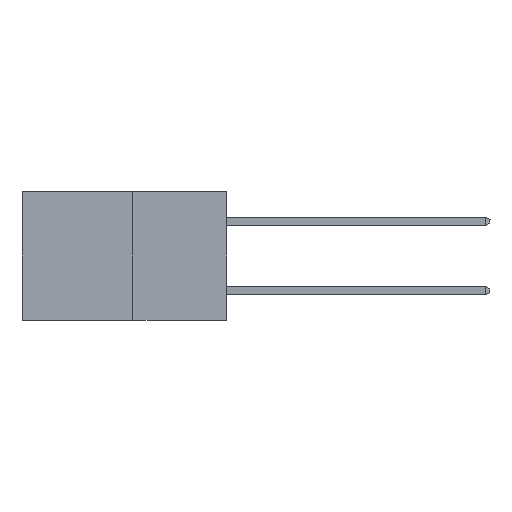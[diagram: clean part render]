
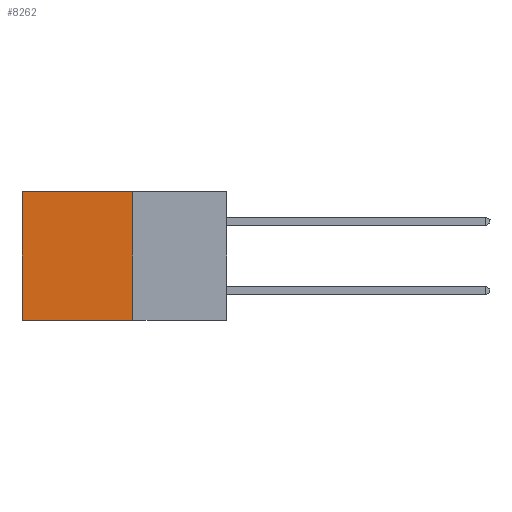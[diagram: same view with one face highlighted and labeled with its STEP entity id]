
A CAD part, left-side view. The second image highlights one B-rep face of the part: STEP entity #8262.
In plain terms, the highlighted planar face has unit normal (-1, 0, 0).
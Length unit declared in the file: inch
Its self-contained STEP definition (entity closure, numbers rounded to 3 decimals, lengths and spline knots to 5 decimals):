
#86 = ORIENTED_EDGE ( 'NONE', *, *, #1455, .T. ) ;
#117 = ORIENTED_EDGE ( 'NONE', *, *, #8861, .F. ) ;
#128 = ORIENTED_EDGE ( 'NONE', *, *, #6020, .F. ) ;
#151 = ORIENTED_EDGE ( 'NONE', *, *, #6541, .T. ) ;
#422 = DIRECTION ( 'NONE',  ( 0., 0., -1. ) ) ;
#516 = CARTESIAN_POINT ( 'NONE',  ( 0.277, 0.59, -0.37 ) ) ;
#811 = FACE_OUTER_BOUND ( 'NONE', #1362, .T. ) ;
#1362 = EDGE_LOOP ( 'NONE', ( #86, #117, #128, #151 ) ) ;
#1455 = EDGE_CURVE ( 'NONE', #7280, #6824, #5242, .T. ) ;
#1714 = CARTESIAN_POINT ( 'NONE',  ( 0.277, 0.27, -0.37 ) ) ;
#1797 = VERTEX_POINT ( 'NONE', #8245 ) ;
#2055 = LINE ( 'NONE', #5171, #2312 ) ;
#2056 = VERTEX_POINT ( 'NONE', #5790 ) ;
#2312 = VECTOR ( 'NONE', #7397, 39.37008 ) ;
#2597 = CARTESIAN_POINT ( 'NONE',  ( 0.277, 0.27, -0.37 ) ) ;
#3045 = DIRECTION ( 'NONE',  ( 0., 1., 0. ) ) ;
#3148 = VECTOR ( 'NONE', #422, 39.37008 ) ;
#3418 = DIRECTION ( 'NONE',  ( 0., 0., -1. ) ) ;
#4685 = LINE ( 'NONE', #1714, #8366 ) ;
#5171 = CARTESIAN_POINT ( 'NONE',  ( 0.277, 0.27, -0.37 ) ) ;
#5242 = LINE ( 'NONE', #516, #3148 ) ;
#5641 = VECTOR ( 'NONE', #3045, 39.37008 ) ;
#5790 = CARTESIAN_POINT ( 'NONE',  ( 0.277, 0.27, -0.37 ) ) ;
#6020 = EDGE_CURVE ( 'NONE', #1797, #2056, #2055, .T. ) ;
#6074 = CARTESIAN_POINT ( 'NONE',  ( 0.277, 0.59, 0. ) ) ;
#6541 = EDGE_CURVE ( 'NONE', #1797, #7280, #7398, .T. ) ;
#6824 = VERTEX_POINT ( 'NONE', #9895 ) ;
#7195 = DIRECTION ( 'NONE',  ( 0., 1., 0. ) ) ;
#7236 = PLANE ( 'NONE',  #8304 ) ;
#7280 = VERTEX_POINT ( 'NONE', #6074 ) ;
#7397 = DIRECTION ( 'NONE',  ( 0., 0., -1. ) ) ;
#7398 = LINE ( 'NONE', #7616, #5641 ) ;
#7616 = CARTESIAN_POINT ( 'NONE',  ( 0.277, 0.27, 0. ) ) ;
#7960 = DIRECTION ( 'NONE',  ( 1., 0., 0. ) ) ;
#8245 = CARTESIAN_POINT ( 'NONE',  ( 0.277, 0.27, 0. ) ) ;
#8262 = ADVANCED_FACE ( 'NONE', ( #811 ), #7236, .F. ) ;
#8304 = AXIS2_PLACEMENT_3D ( 'NONE', #2597, #7960, #3418 ) ;
#8366 = VECTOR ( 'NONE', #7195, 39.37008 ) ;
#8861 = EDGE_CURVE ( 'NONE', #2056, #6824, #4685, .T. ) ;
#9895 = CARTESIAN_POINT ( 'NONE',  ( 0.277, 0.59, -0.37 ) ) ;
